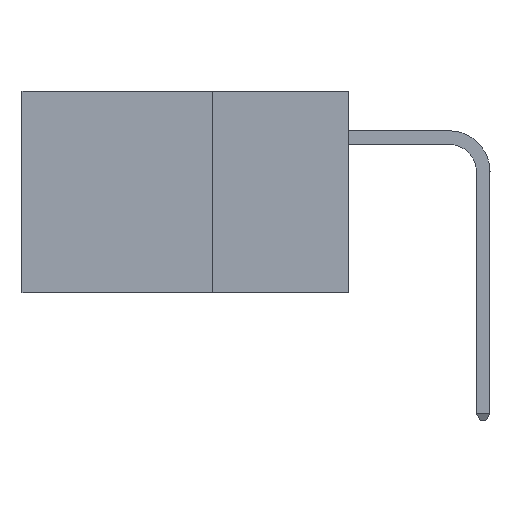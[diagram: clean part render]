
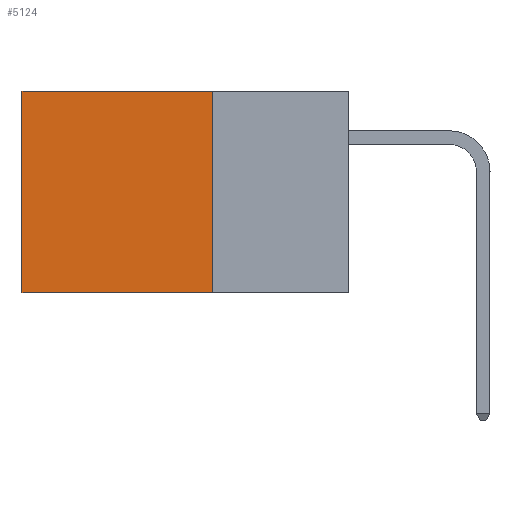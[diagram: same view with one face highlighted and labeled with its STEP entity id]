
A CAD part, left-side view. The second image highlights one B-rep face of the part: STEP entity #5124.
In plain terms, the highlighted planar face has unit normal (-1, 0, 0).
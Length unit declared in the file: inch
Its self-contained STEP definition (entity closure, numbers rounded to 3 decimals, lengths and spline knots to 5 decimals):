
#1299 = CARTESIAN_POINT ( 'NONE',  ( 0.2875, 0.25, 0. ) ) ;
#2405 = LINE ( 'NONE', #5473, #25232 ) ;
#2792 = VERTEX_POINT ( 'NONE', #22041 ) ;
#3572 = DIRECTION ( 'NONE',  ( 0., 1., 0. ) ) ;
#3897 = ORIENTED_EDGE ( 'NONE', *, *, #13659, .T. ) ;
#4361 = CARTESIAN_POINT ( 'NONE',  ( 0.2875, 0.25, 0. ) ) ;
#4586 = EDGE_CURVE ( 'NONE', #7611, #13043, #11654, .T. ) ;
#5124 = ADVANCED_FACE ( 'NONE', ( #26285 ), #18652, .F. ) ;
#5335 = DIRECTION ( 'NONE',  ( 1., 0., 0. ) ) ;
#5473 = CARTESIAN_POINT ( 'NONE',  ( 0.2875, 0.25, -0.37 ) ) ;
#6629 = LINE ( 'NONE', #14589, #18484 ) ;
#7611 = VERTEX_POINT ( 'NONE', #4361 ) ;
#9025 = EDGE_LOOP ( 'NONE', ( #3897, #24835, #12354, #23478 ) ) ;
#9232 = EDGE_CURVE ( 'NONE', #13438, #2792, #2405, .T. ) ;
#9390 = AXIS2_PLACEMENT_3D ( 'NONE', #16444, #5335, #20818 ) ;
#10118 = DIRECTION ( 'NONE',  ( 0., 0., -1. ) ) ;
#11654 = LINE ( 'NONE', #1299, #28361 ) ;
#12354 = ORIENTED_EDGE ( 'NONE', *, *, #26037, .F. ) ;
#13043 = VERTEX_POINT ( 'NONE', #19038 ) ;
#13438 = VERTEX_POINT ( 'NONE', #22540 ) ;
#13659 = EDGE_CURVE ( 'NONE', #13043, #2792, #24615, .T. ) ;
#14589 = CARTESIAN_POINT ( 'NONE',  ( 0.2875, 0.25, 0. ) ) ;
#16444 = CARTESIAN_POINT ( 'NONE',  ( 0.2875, 0.25, 0. ) ) ;
#18484 = VECTOR ( 'NONE', #23272, 39.37008 ) ;
#18652 = PLANE ( 'NONE',  #9390 ) ;
#19038 = CARTESIAN_POINT ( 'NONE',  ( 0.2875, 0.6, 0. ) ) ;
#20818 = DIRECTION ( 'NONE',  ( 0., 0., -1. ) ) ;
#21094 = CARTESIAN_POINT ( 'NONE',  ( 0.2875, 0.6, 0. ) ) ;
#22041 = CARTESIAN_POINT ( 'NONE',  ( 0.2875, 0.6, -0.37 ) ) ;
#22540 = CARTESIAN_POINT ( 'NONE',  ( 0.2875, 0.25, -0.37 ) ) ;
#23149 = DIRECTION ( 'NONE',  ( 0., 1., 0. ) ) ;
#23272 = DIRECTION ( 'NONE',  ( 0., 0., -1. ) ) ;
#23478 = ORIENTED_EDGE ( 'NONE', *, *, #4586, .T. ) ;
#23944 = VECTOR ( 'NONE', #10118, 39.37008 ) ;
#24615 = LINE ( 'NONE', #21094, #23944 ) ;
#24835 = ORIENTED_EDGE ( 'NONE', *, *, #9232, .F. ) ;
#25232 = VECTOR ( 'NONE', #23149, 39.37008 ) ;
#26037 = EDGE_CURVE ( 'NONE', #7611, #13438, #6629, .T. ) ;
#26285 = FACE_OUTER_BOUND ( 'NONE', #9025, .T. ) ;
#28361 = VECTOR ( 'NONE', #3572, 39.37008 ) ;
